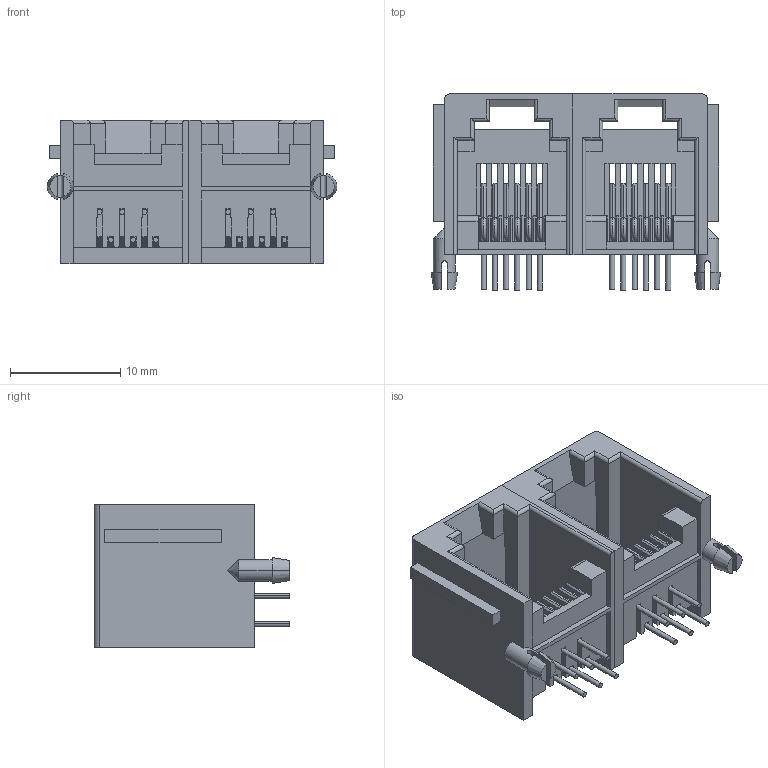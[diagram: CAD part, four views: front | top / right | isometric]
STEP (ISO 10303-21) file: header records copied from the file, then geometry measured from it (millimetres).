
FILE_DESCRIPTION (( 'STEP AP203' ), '1' );
FILE_NAME ('RJ53026692N00013.STEP', '2020-01-08T16:20:00', ( '' ), ( '' ), 'SwSTEP 2.0', 'SolidWorks 2016', '' );
FILE_SCHEMA (( 'CONFIG_CONTROL_DESIGN' ));
Length unit declared in the file: millimetre
Products named in the file (10): 53 Contact - 1; 53 Contact - 4; 53 Contact - 3; 53 Contact - 2; 53 Contacts; 53 Insulator LH; 53 Contact - 5; 53 Insulator RH; 53 Contact - 6; RJ53026692N00013
Assembly tree (10 placements, depth 3):
  RJ53026692N00013
    53 Insulator RH
    53 Insulator LH
    53 Contacts  x2
      53 Contact - 6
      53 Contact - 4
      53 Contact - 2
      53 Contact - 5
      53 Contact - 3
      53 Contact - 1
Bounding box: 26.25 x 17.75 x 13 mm (x, y, z)
Volume: 1800.2 mm3; surface area: 4280.4 mm2
Topology: 14 solids, 14 shells, 595 faces, 1664 edges, 1058 vertices
Faces by surface type: plane 410, cylinder 128, torus 48, cone 9
Entity records: 18147 total; most frequent: CARTESIAN_POINT 3184, ORIENTED_EDGE 3034, DIRECTION 2735, EDGE_CURVE 1517, LINE 1285, VECTOR 1285, VERTEX_POINT 974, AXIS2_PLACEMENT_3D 725
